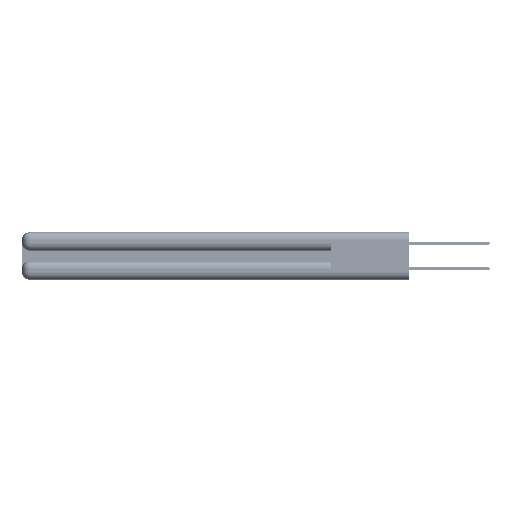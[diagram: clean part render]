
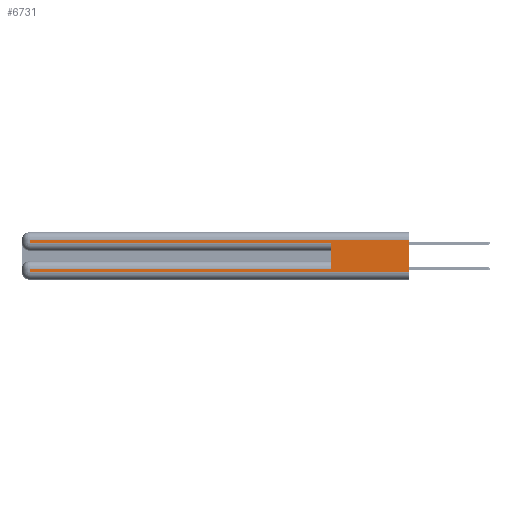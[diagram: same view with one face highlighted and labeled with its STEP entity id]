
A CAD part, left-side view. The second image highlights one B-rep face of the part: STEP entity #6731.
In plain terms, the highlighted planar face has unit normal (-1, 0, 0).
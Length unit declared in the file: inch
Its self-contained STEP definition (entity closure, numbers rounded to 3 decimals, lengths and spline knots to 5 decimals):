
#679 = CARTESIAN_POINT ( 'NONE',  ( 0., 0.6, 0.285 ) ) ;
#865 = VERTEX_POINT ( 'NONE', #679 ) ;
#1052 = CARTESIAN_POINT ( 'NONE',  ( 0., 0.6, 0.085 ) ) ;
#1191 = VECTOR ( 'NONE', #43978, 39.37008 ) ;
#1782 = VERTEX_POINT ( 'NONE', #27366 ) ;
#2323 = DIRECTION ( 'NONE',  ( 0., 0., -1. ) ) ;
#2913 = CARTESIAN_POINT ( 'NONE',  ( 0., 0., 0.37 ) ) ;
#4019 = VECTOR ( 'NONE', #2323, 39.37008 ) ;
#5400 = VECTOR ( 'NONE', #48557, 39.37008 ) ;
#5529 = VERTEX_POINT ( 'NONE', #43775 ) ;
#5685 = EDGE_CURVE ( 'NONE', #36352, #47619, #9344, .T. ) ;
#6173 = ORIENTED_EDGE ( 'NONE', *, *, #15752, .F. ) ;
#6572 = VECTOR ( 'NONE', #44082, 39.37008 ) ;
#6731 = ADVANCED_FACE ( 'NONE', ( #20360 ), #6875, .F. ) ;
#6875 = PLANE ( 'NONE',  #37459 ) ;
#7013 = CARTESIAN_POINT ( 'NONE',  ( 0., 0.6, 0.145 ) ) ;
#7051 = DIRECTION ( 'NONE',  ( 0., 0., -1. ) ) ;
#7399 = CARTESIAN_POINT ( 'NONE',  ( 0., 2.94, 0.31 ) ) ;
#8194 = EDGE_CURVE ( 'NONE', #8846, #1782, #38164, .T. ) ;
#8846 = VERTEX_POINT ( 'NONE', #7399 ) ;
#9344 = LINE ( 'NONE', #24204, #42096 ) ;
#9638 = LINE ( 'NONE', #29076, #20593 ) ;
#10104 = EDGE_CURVE ( 'NONE', #40008, #8846, #12237, .T. ) ;
#11210 = ORIENTED_EDGE ( 'NONE', *, *, #8194, .T. ) ;
#12177 = EDGE_CURVE ( 'NONE', #50913, #865, #44843, .T. ) ;
#12237 = LINE ( 'NONE', #15386, #34076 ) ;
#13868 = CARTESIAN_POINT ( 'NONE',  ( 0., 0., 0.31 ) ) ;
#15386 = CARTESIAN_POINT ( 'NONE',  ( 0., 0., 0.31 ) ) ;
#15752 = EDGE_CURVE ( 'NONE', #40008, #47619, #9638, .T. ) ;
#17155 = CARTESIAN_POINT ( 'NONE',  ( 0., 2.94, 0.06 ) ) ;
#20360 = FACE_OUTER_BOUND ( 'NONE', #38206, .T. ) ;
#20593 = VECTOR ( 'NONE', #41456, 39.37008 ) ;
#23646 = CARTESIAN_POINT ( 'NONE',  ( 0., 0., 0.085 ) ) ;
#24204 = CARTESIAN_POINT ( 'NONE',  ( 0., 0., 0.06 ) ) ;
#25219 = ORIENTED_EDGE ( 'NONE', *, *, #12177, .F. ) ;
#27163 = LINE ( 'NONE', #39123, #4019 ) ;
#27366 = CARTESIAN_POINT ( 'NONE',  ( 0., 2.94, 0.285 ) ) ;
#28866 = CARTESIAN_POINT ( 'NONE',  ( 0., 0., 0.285 ) ) ;
#29076 = CARTESIAN_POINT ( 'NONE',  ( 0., 0., 0.37 ) ) ;
#29206 = EDGE_CURVE ( 'NONE', #50913, #5529, #39327, .T. ) ;
#29385 = CARTESIAN_POINT ( 'NONE',  ( 0., 0., 0.06 ) ) ;
#29857 = ORIENTED_EDGE ( 'NONE', *, *, #10104, .T. ) ;
#31641 = DIRECTION ( 'NONE',  ( 1., 0., 0. ) ) ;
#32990 = DIRECTION ( 'NONE',  ( 0., -1., 0. ) ) ;
#34076 = VECTOR ( 'NONE', #44063, 39.37008 ) ;
#35551 = ORIENTED_EDGE ( 'NONE', *, *, #5685, .T. ) ;
#36352 = VERTEX_POINT ( 'NONE', #17155 ) ;
#37459 = AXIS2_PLACEMENT_3D ( 'NONE', #2913, #31641, #7051 ) ;
#38164 = LINE ( 'NONE', #52652, #5400 ) ;
#38206 = EDGE_LOOP ( 'NONE', ( #6173, #29857, #11210, #51412, #25219, #46092, #47732, #35551 ) ) ;
#39123 = CARTESIAN_POINT ( 'NONE',  ( 0., 2.94, 0.37 ) ) ;
#39327 = LINE ( 'NONE', #23646, #6572 ) ;
#40008 = VERTEX_POINT ( 'NONE', #13868 ) ;
#40974 = EDGE_CURVE ( 'NONE', #1782, #865, #41472, .T. ) ;
#41456 = DIRECTION ( 'NONE',  ( 0., 0., -1. ) ) ;
#41472 = LINE ( 'NONE', #28866, #42756 ) ;
#42096 = VECTOR ( 'NONE', #52864, 39.37008 ) ;
#42720 = EDGE_CURVE ( 'NONE', #5529, #36352, #27163, .T. ) ;
#42756 = VECTOR ( 'NONE', #32990, 39.37008 ) ;
#43775 = CARTESIAN_POINT ( 'NONE',  ( 0., 2.94, 0.085 ) ) ;
#43978 = DIRECTION ( 'NONE',  ( 0., 0., 1. ) ) ;
#44063 = DIRECTION ( 'NONE',  ( 0., 1., 0. ) ) ;
#44082 = DIRECTION ( 'NONE',  ( 0., 1., 0. ) ) ;
#44843 = LINE ( 'NONE', #7013, #1191 ) ;
#46092 = ORIENTED_EDGE ( 'NONE', *, *, #29206, .T. ) ;
#47619 = VERTEX_POINT ( 'NONE', #29385 ) ;
#47732 = ORIENTED_EDGE ( 'NONE', *, *, #42720, .T. ) ;
#48557 = DIRECTION ( 'NONE',  ( 0., 0., -1. ) ) ;
#50913 = VERTEX_POINT ( 'NONE', #1052 ) ;
#51412 = ORIENTED_EDGE ( 'NONE', *, *, #40974, .T. ) ;
#52652 = CARTESIAN_POINT ( 'NONE',  ( 0., 2.94, 0.37 ) ) ;
#52864 = DIRECTION ( 'NONE',  ( 0., -1., 0. ) ) ;
